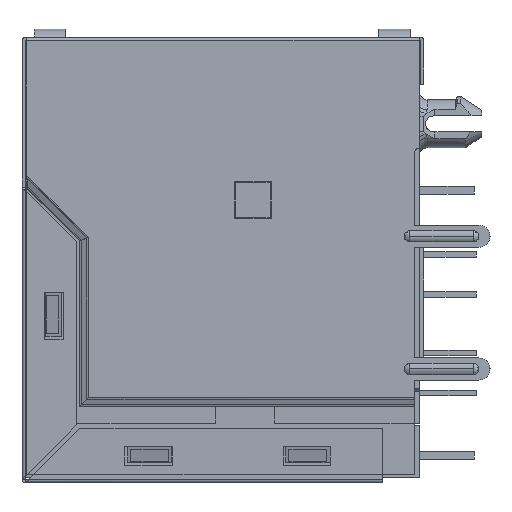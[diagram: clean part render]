
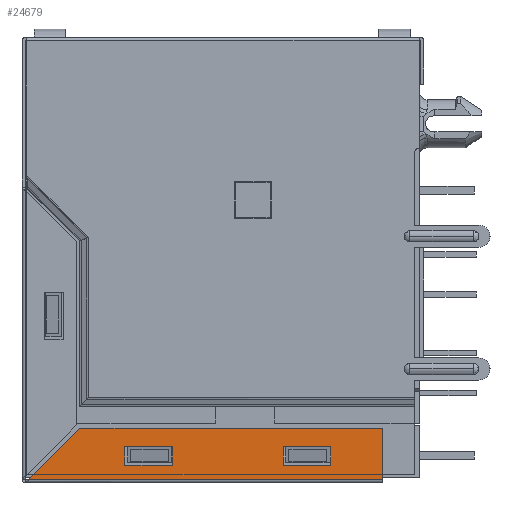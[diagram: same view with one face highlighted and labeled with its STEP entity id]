
A CAD part, left-side view. The second image highlights one B-rep face of the part: STEP entity #24679.
In plain terms, the highlighted planar face has unit normal (-1, 0, 0).
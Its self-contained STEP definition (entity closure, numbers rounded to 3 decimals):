
#1544 = ORIENTED_EDGE ( 'NONE', *, *, #40101, .F. ) ;
#3483 = CARTESIAN_POINT ( 'NONE',  ( -31.875, 3.165, -26.78 ) ) ;
#5843 = CARTESIAN_POINT ( 'NONE',  ( -31.875, 12.245, -27.67 ) ) ;
#7179 = CARTESIAN_POINT ( 'NONE',  ( -31.875, 12.245, -27.67 ) ) ;
#9991 = ORIENTED_EDGE ( 'NONE', *, *, #56747, .T. ) ;
#11469 = CARTESIAN_POINT ( 'NONE',  ( -31.875, 9.005, -24.43 ) ) ;
#12052 = EDGE_CURVE ( 'NONE', #134280, #80826, #74557, .T. ) ;
#14128 = FACE_BOUND ( 'NONE', #75239, .T. ) ;
#15333 = CARTESIAN_POINT ( 'NONE',  ( -31.875, -10.135, -27.67 ) ) ;
#15365 = EDGE_CURVE ( 'NONE', #80826, #129101, #139096, .T. ) ;
#16029 = CARTESIAN_POINT ( 'NONE',  ( -31.875, -3.835, -26.78 ) ) ;
#16993 = ORIENTED_EDGE ( 'NONE', *, *, #105747, .T. ) ;
#21979 = CARTESIAN_POINT ( 'NONE',  ( -31.875, -6.835, -25.58 ) ) ;
#23200 = VERTEX_POINT ( 'NONE', #23264 ) ;
#23264 = CARTESIAN_POINT ( 'NONE',  ( -31.875, -6.835, -25.58 ) ) ;
#23646 = ORIENTED_EDGE ( 'NONE', *, *, #31978, .T. ) ;
#23948 = CARTESIAN_POINT ( 'NONE',  ( -31.875, 3.165, -25.58 ) ) ;
#24679 = ADVANCED_FACE ( 'NONE', ( #72788, #14128, #34929 ), #34952, .T. ) ;
#24723 = CARTESIAN_POINT ( 'NONE',  ( -31.875, -10.135, -24.43 ) ) ;
#27558 = CARTESIAN_POINT ( 'NONE',  ( -31.875, 9.005, -24.43 ) ) ;
#31978 = EDGE_CURVE ( 'NONE', #43655, #103167, #80588, .T. ) ;
#34826 = CARTESIAN_POINT ( 'NONE',  ( -31.875, 6.165, -25.58 ) ) ;
#34929 = FACE_BOUND ( 'NONE', #50408, .T. ) ;
#34952 = PLANE ( 'NONE',  #122382 ) ;
#35408 = VERTEX_POINT ( 'NONE', #34826 ) ;
#37531 = CARTESIAN_POINT ( 'NONE',  ( -31.875, -10.135, -24.43 ) ) ;
#38615 = CARTESIAN_POINT ( 'NONE',  ( -31.875, 6.165, -25.58 ) ) ;
#40101 = EDGE_CURVE ( 'NONE', #74898, #134280, #122253, .T. ) ;
#43655 = VERTEX_POINT ( 'NONE', #23948 ) ;
#44106 = ORIENTED_EDGE ( 'NONE', *, *, #15365, .F. ) ;
#45240 = CARTESIAN_POINT ( 'NONE',  ( -31.875, -10.135, -24.43 ) ) ;
#45675 = ORIENTED_EDGE ( 'NONE', *, *, #134124, .T. ) ;
#46753 = ORIENTED_EDGE ( 'NONE', *, *, #12052, .F. ) ;
#47105 = EDGE_CURVE ( 'NONE', #74898, #129101, #52382, .T. ) ;
#50408 = EDGE_LOOP ( 'NONE', ( #53000, #16993, #108057, #45675 ) ) ;
#50438 = CARTESIAN_POINT ( 'NONE',  ( -31.875, 6.165, -26.78 ) ) ;
#51086 = B_SPLINE_CURVE_WITH_KNOTS ( 'NONE', 1,
 ( #140162, #63391 ),
 .UNSPECIFIED., .F., .F.,
 ( 2, 2 ),
 ( 0., 1. ),
 .UNSPECIFIED. ) ;
#52028 = ORIENTED_EDGE ( 'NONE', *, *, #111900, .T. ) ;
#52382 = B_SPLINE_CURVE_WITH_KNOTS ( 'NONE', 1,
 ( #118772, #108637 ),
 .UNSPECIFIED., .F., .F.,
 ( 2, 2 ),
 ( 0., 1. ),
 .UNSPECIFIED. ) ;
#52431 = CARTESIAN_POINT ( 'NONE',  ( -31.875, -3.835, -26.78 ) ) ;
#53000 = ORIENTED_EDGE ( 'NONE', *, *, #137132, .T. ) ;
#53045 = CARTESIAN_POINT ( 'NONE',  ( -31.875, 3.165, -25.58 ) ) ;
#56747 = EDGE_CURVE ( 'NONE', #89695, #35408, #90198, .T. ) ;
#60224 = ORIENTED_EDGE ( 'NONE', *, *, #47105, .T. ) ;
#63391 = CARTESIAN_POINT ( 'NONE',  ( -31.875, 3.165, -25.58 ) ) ;
#64090 = CARTESIAN_POINT ( 'NONE',  ( -31.875, 3.165, -26.78 ) ) ;
#64423 = CARTESIAN_POINT ( 'NONE',  ( -31.875, -3.835, -25.58 ) ) ;
#64491 = CARTESIAN_POINT ( 'NONE',  ( -31.875, -6.835, -26.78 ) ) ;
#68058 = B_SPLINE_CURVE_WITH_KNOTS ( 'NONE', 1,
 ( #125709, #126190 ),
 .UNSPECIFIED., .F., .F.,
 ( 2, 2 ),
 ( 0., 1. ),
 .UNSPECIFIED. ) ;
#68159 = CARTESIAN_POINT ( 'NONE',  ( -31.875, 12.693, -27.766 ) ) ;
#71457 = CARTESIAN_POINT ( 'NONE',  ( -31.875, -6.835, -26.78 ) ) ;
#72788 = FACE_OUTER_BOUND ( 'NONE', #85188, .T. ) ;
#74557 = B_SPLINE_CURVE_WITH_KNOTS ( 'NONE', 1,
 ( #11469, #45240 ),
 .UNSPECIFIED., .F., .F.,
 ( 2, 2 ),
 ( 0., 1. ),
 .UNSPECIFIED. ) ;
#74898 = VERTEX_POINT ( 'NONE', #7179 ) ;
#75239 = EDGE_LOOP ( 'NONE', ( #9991, #52028, #23646, #109252 ) ) ;
#75683 = CARTESIAN_POINT ( 'NONE',  ( -31.875, -10.135, -27.67 ) ) ;
#77171 = VERTEX_POINT ( 'NONE', #133350 ) ;
#80588 = B_SPLINE_CURVE_WITH_KNOTS ( 'NONE', 1,
 ( #53045, #64090 ),
 .UNSPECIFIED., .F., .F.,
 ( 2, 2 ),
 ( 0., 1. ),
 .UNSPECIFIED. ) ;
#80826 = VERTEX_POINT ( 'NONE', #24723 ) ;
#85188 = EDGE_LOOP ( 'NONE', ( #1544, #60224, #44106, #46753 ) ) ;
#89105 = B_SPLINE_CURVE_WITH_KNOTS ( 'NONE', 1,
 ( #131957, #21979 ),
 .UNSPECIFIED., .F., .F.,
 ( 2, 2 ),
 ( 0., 1. ),
 .UNSPECIFIED. ) ;
#89650 = EDGE_CURVE ( 'NONE', #103167, #89695, #68058, .T. ) ;
#89695 = VERTEX_POINT ( 'NONE', #50438 ) ;
#90198 = B_SPLINE_CURVE_WITH_KNOTS ( 'NONE', 1,
 ( #94495, #38615 ),
 .UNSPECIFIED., .F., .F.,
 ( 2, 2 ),
 ( 0., 1. ),
 .UNSPECIFIED. ) ;
#91780 = DIRECTION ( 'NONE',  ( -1., 0., 0. ) ) ;
#94495 = CARTESIAN_POINT ( 'NONE',  ( -31.875, 6.165, -26.78 ) ) ;
#96493 = CARTESIAN_POINT ( 'NONE',  ( -31.875, 9.005, -24.43 ) ) ;
#99767 = VERTEX_POINT ( 'NONE', #129450 ) ;
#103167 = VERTEX_POINT ( 'NONE', #3483 ) ;
#105747 = EDGE_CURVE ( 'NONE', #99767, #23200, #89105, .T. ) ;
#107540 = VERTEX_POINT ( 'NONE', #126904 ) ;
#107876 = CARTESIAN_POINT ( 'NONE',  ( -31.875, -6.835, -25.58 ) ) ;
#108057 = ORIENTED_EDGE ( 'NONE', *, *, #129443, .T. ) ;
#108637 = CARTESIAN_POINT ( 'NONE',  ( -31.875, -10.135, -27.67 ) ) ;
#109252 = ORIENTED_EDGE ( 'NONE', *, *, #89650, .T. ) ;
#111900 = EDGE_CURVE ( 'NONE', #35408, #43655, #51086, .T. ) ;
#117189 = B_SPLINE_CURVE_WITH_KNOTS ( 'NONE', 1,
 ( #52431, #64423 ),
 .UNSPECIFIED., .F., .F.,
 ( 2, 2 ),
 ( 0., 1. ),
 .UNSPECIFIED. ) ;
#118772 = CARTESIAN_POINT ( 'NONE',  ( -31.875, 12.245, -27.67 ) ) ;
#122253 = B_SPLINE_CURVE_WITH_KNOTS ( 'NONE', 1,
 ( #5843, #27558 ),
 .UNSPECIFIED., .F., .F.,
 ( 2, 2 ),
 ( 0., 1. ),
 .UNSPECIFIED. ) ;
#122382 = AXIS2_PLACEMENT_3D ( 'NONE', #68159, #91780, #135208 ) ;
#123595 = B_SPLINE_CURVE_WITH_KNOTS ( 'NONE', 1,
 ( #71457, #16029 ),
 .UNSPECIFIED., .F., .F.,
 ( 2, 2 ),
 ( 0., 1. ),
 .UNSPECIFIED. ) ;
#124589 = B_SPLINE_CURVE_WITH_KNOTS ( 'NONE', 1,
 ( #107876, #64491 ),
 .UNSPECIFIED., .F., .F.,
 ( 2, 2 ),
 ( 0., 1. ),
 .UNSPECIFIED. ) ;
#125709 = CARTESIAN_POINT ( 'NONE',  ( -31.875, 3.165, -26.78 ) ) ;
#126190 = CARTESIAN_POINT ( 'NONE',  ( -31.875, 6.165, -26.78 ) ) ;
#126904 = CARTESIAN_POINT ( 'NONE',  ( -31.875, -3.835, -26.78 ) ) ;
#129101 = VERTEX_POINT ( 'NONE', #75683 ) ;
#129443 = EDGE_CURVE ( 'NONE', #23200, #77171, #124589, .T. ) ;
#129450 = CARTESIAN_POINT ( 'NONE',  ( -31.875, -3.835, -25.58 ) ) ;
#131957 = CARTESIAN_POINT ( 'NONE',  ( -31.875, -3.835, -25.58 ) ) ;
#133350 = CARTESIAN_POINT ( 'NONE',  ( -31.875, -6.835, -26.78 ) ) ;
#134124 = EDGE_CURVE ( 'NONE', #77171, #107540, #123595, .T. ) ;
#134280 = VERTEX_POINT ( 'NONE', #96493 ) ;
#135208 = DIRECTION ( 'NONE',  ( 0., -1., 0. ) ) ;
#137132 = EDGE_CURVE ( 'NONE', #107540, #99767, #117189, .T. ) ;
#139096 = B_SPLINE_CURVE_WITH_KNOTS ( 'NONE', 1,
 ( #37531, #15333 ),
 .UNSPECIFIED., .F., .F.,
 ( 2, 2 ),
 ( 0., 1. ),
 .UNSPECIFIED. ) ;
#140162 = CARTESIAN_POINT ( 'NONE',  ( -31.875, 6.165, -25.58 ) ) ;
